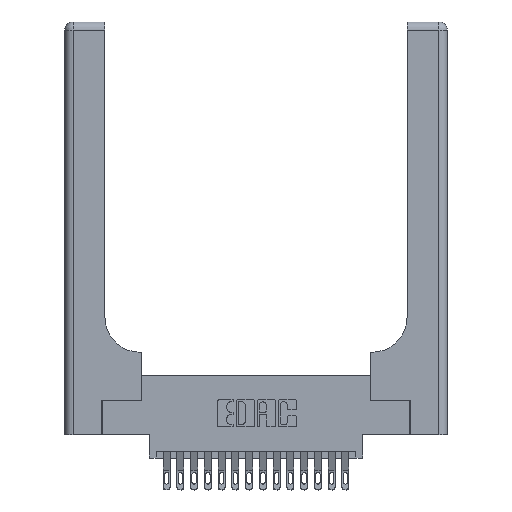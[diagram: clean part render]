
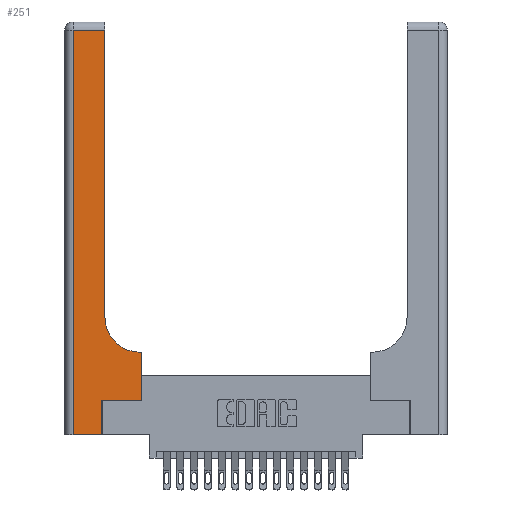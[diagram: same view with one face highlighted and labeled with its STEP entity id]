
A CAD part, top view. The second image highlights one B-rep face of the part: STEP entity #251.
In plain terms, the highlighted planar face has unit normal (0, 0, 1).
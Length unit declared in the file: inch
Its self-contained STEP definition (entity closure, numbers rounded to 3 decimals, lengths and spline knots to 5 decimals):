
#251 = ADVANCED_FACE ( 'NONE', ( #9278 ), #6512, .F. ) ;
#450 = DIRECTION ( 'NONE',  ( 1., 0., 0. ) ) ;
#748 = EDGE_CURVE ( 'NONE', #9908, #10132, #17522, .T. ) ;
#771 = CARTESIAN_POINT ( 'NONE',  ( 0.2915, 3., 0.37 ) ) ;
#1830 = EDGE_CURVE ( 'NONE', #13548, #10981, #15114, .T. ) ;
#2218 = VECTOR ( 'NONE', #2390, 39.37008 ) ;
#2390 = DIRECTION ( 'NONE',  ( 0., 1., 0. ) ) ;
#2609 = VERTEX_POINT ( 'NONE', #13878 ) ;
#3724 = CARTESIAN_POINT ( 'NONE',  ( 0., 2.94, 0.37 ) ) ;
#4007 = EDGE_CURVE ( 'NONE', #5542, #9908, #5035, .T. ) ;
#4133 = LINE ( 'NONE', #14375, #9015 ) ;
#5035 = LINE ( 'NONE', #19948, #17657 ) ;
#5069 = EDGE_CURVE ( 'NONE', #9038, #13548, #8897, .T. ) ;
#5542 = VERTEX_POINT ( 'NONE', #18931 ) ;
#5841 = DIRECTION ( 'NONE',  ( -1., 0., 0. ) ) ;
#5853 = DIRECTION ( 'NONE',  ( 0., -1., 0. ) ) ;
#5865 = DIRECTION ( 'NONE',  ( 0., 0., -1. ) ) ;
#5906 = CARTESIAN_POINT ( 'NONE',  ( 0.06, 3., 0.37 ) ) ;
#6274 = CARTESIAN_POINT ( 'NONE',  ( 0., 3., 0.37 ) ) ;
#6450 = EDGE_CURVE ( 'NONE', #10132, #9038, #19004, .T. ) ;
#6512 = PLANE ( 'NONE',  #16393 ) ;
#6634 = VECTOR ( 'NONE', #5853, 39.37008 ) ;
#6745 = CARTESIAN_POINT ( 'NONE',  ( 0.5585, 0.25, 0.37 ) ) ;
#7171 = ORIENTED_EDGE ( 'NONE', *, *, #6450, .T. ) ;
#7216 = ORIENTED_EDGE ( 'NONE', *, *, #5069, .T. ) ;
#7348 = ORIENTED_EDGE ( 'NONE', *, *, #1830, .T. ) ;
#7365 = ORIENTED_EDGE ( 'NONE', *, *, #9631, .T. ) ;
#7500 = ORIENTED_EDGE ( 'NONE', *, *, #8942, .T. ) ;
#7532 = VECTOR ( 'NONE', #16233, 39.37008 ) ;
#7547 = ORIENTED_EDGE ( 'NONE', *, *, #14000, .T. ) ;
#7645 = ORIENTED_EDGE ( 'NONE', *, *, #8236, .T. ) ;
#7720 = ORIENTED_EDGE ( 'NONE', *, *, #4007, .T. ) ;
#7782 = ORIENTED_EDGE ( 'NONE', *, *, #748, .T. ) ;
#8236 = EDGE_CURVE ( 'NONE', #8844, #5542, #18969, .T. ) ;
#8539 = CARTESIAN_POINT ( 'NONE',  ( 0.269, 0.25, 0.37 ) ) ;
#8844 = VERTEX_POINT ( 'NONE', #6745 ) ;
#8897 = LINE ( 'NONE', #3724, #16229 ) ;
#8942 = EDGE_CURVE ( 'NONE', #2609, #14007, #16121, .T. ) ;
#9015 = VECTOR ( 'NONE', #17438, 39.37008 ) ;
#9038 = VERTEX_POINT ( 'NONE', #9040 ) ;
#9040 = CARTESIAN_POINT ( 'NONE',  ( 0.2915, 2.94, 0.37 ) ) ;
#9278 = FACE_OUTER_BOUND ( 'NONE', #11512, .T. ) ;
#9631 = EDGE_CURVE ( 'NONE', #10981, #2609, #4133, .T. ) ;
#9805 = VECTOR ( 'NONE', #450, 39.37008 ) ;
#9908 = VERTEX_POINT ( 'NONE', #19502 ) ;
#10132 = VERTEX_POINT ( 'NONE', #19945 ) ;
#10252 = CARTESIAN_POINT ( 'NONE',  ( 0.269, 0., 0.37 ) ) ;
#10437 = AXIS2_PLACEMENT_3D ( 'NONE', #15395, #15319, #15203 ) ;
#10981 = VERTEX_POINT ( 'NONE', #11605 ) ;
#11512 = EDGE_LOOP ( 'NONE', ( #7171, #7216, #7348, #7365, #7500, #7547, #7645, #7720, #7782 ) ) ;
#11605 = CARTESIAN_POINT ( 'NONE',  ( 0.06, 0., 0.37 ) ) ;
#11790 = CARTESIAN_POINT ( 'NONE',  ( 0.269, 0.25, 0.37 ) ) ;
#11853 = DIRECTION ( 'NONE',  ( 0., 1., 0. ) ) ;
#12210 = CARTESIAN_POINT ( 'NONE',  ( 0.06, 2.94, 0.37 ) ) ;
#13548 = VERTEX_POINT ( 'NONE', #12210 ) ;
#13878 = CARTESIAN_POINT ( 'NONE',  ( 0.269, 0., 0.37 ) ) ;
#14000 = EDGE_CURVE ( 'NONE', #14007, #8844, #18029, .T. ) ;
#14007 = VERTEX_POINT ( 'NONE', #11790 ) ;
#14375 = CARTESIAN_POINT ( 'NONE',  ( 0., 0., 0.37 ) ) ;
#14721 = CARTESIAN_POINT ( 'NONE',  ( 0.5585, 0.25, 0.37 ) ) ;
#15114 = LINE ( 'NONE', #5906, #6634 ) ;
#15203 = DIRECTION ( 'NONE',  ( 1., 0., 0. ) ) ;
#15319 = DIRECTION ( 'NONE',  ( 0., 0., -1. ) ) ;
#15395 = CARTESIAN_POINT ( 'NONE',  ( 0.5415, 0.85, 0.37 ) ) ;
#16121 = LINE ( 'NONE', #10252, #16608 ) ;
#16229 = VECTOR ( 'NONE', #16452, 39.37008 ) ;
#16233 = DIRECTION ( 'NONE',  ( 0., 1., 0. ) ) ;
#16393 = AXIS2_PLACEMENT_3D ( 'NONE', #6274, #5865, #5841 ) ;
#16452 = DIRECTION ( 'NONE',  ( -1., 0., 0. ) ) ;
#16608 = VECTOR ( 'NONE', #11853, 39.37008 ) ;
#16902 = DIRECTION ( 'NONE',  ( -1., 0., 0. ) ) ;
#17438 = DIRECTION ( 'NONE',  ( 1., 0., 0. ) ) ;
#17522 = CIRCLE ( 'NONE', #10437, 0.25 ) ;
#17657 = VECTOR ( 'NONE', #16902, 39.37008 ) ;
#18029 = LINE ( 'NONE', #8539, #9805 ) ;
#18931 = CARTESIAN_POINT ( 'NONE',  ( 0.5585, 0.6, 0.37 ) ) ;
#18969 = LINE ( 'NONE', #14721, #7532 ) ;
#19004 = LINE ( 'NONE', #771, #2218 ) ;
#19502 = CARTESIAN_POINT ( 'NONE',  ( 0.5415, 0.6, 0.37 ) ) ;
#19945 = CARTESIAN_POINT ( 'NONE',  ( 0.2915, 0.85, 0.37 ) ) ;
#19948 = CARTESIAN_POINT ( 'NONE',  ( 0.2915, 0.6, 0.37 ) ) ;
